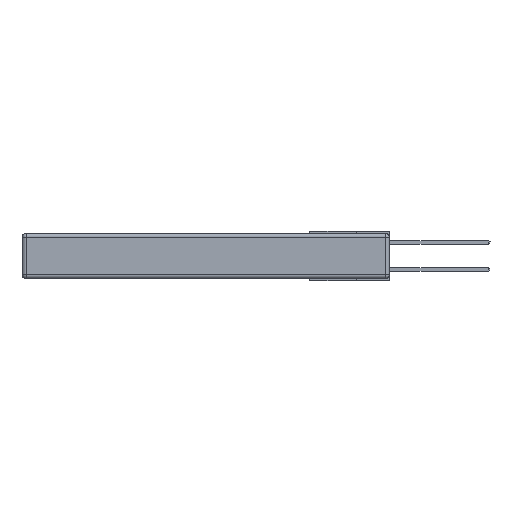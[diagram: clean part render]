
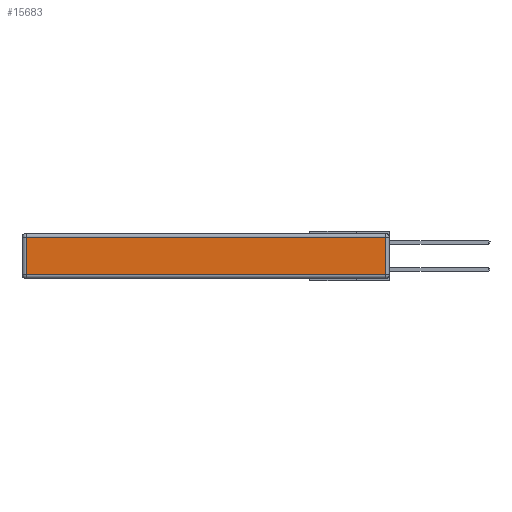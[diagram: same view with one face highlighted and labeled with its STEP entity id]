
A CAD part, left-side view. The second image highlights one B-rep face of the part: STEP entity #15683.
In plain terms, the highlighted planar face has unit normal (-1, 0, 0).
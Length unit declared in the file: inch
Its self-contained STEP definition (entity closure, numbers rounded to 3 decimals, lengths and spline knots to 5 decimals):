
#315 = DIRECTION ( 'NONE',  ( -1., 0., 0. ) ) ;
#1151 = EDGE_CURVE ( 'NONE', #24985, #11487, #11286, .T. ) ;
#1831 = EDGE_LOOP ( 'NONE', ( #15404, #2251, #17438, #33896 ) ) ;
#2251 = ORIENTED_EDGE ( 'NONE', *, *, #24289, .T. ) ;
#4207 = CARTESIAN_POINT ( 'NONE',  ( 0., 0.03, -0.343 ) ) ;
#9116 = VECTOR ( 'NONE', #14674, 39.37008 ) ;
#9779 = CARTESIAN_POINT ( 'NONE',  ( 0., 0.03, -0.313 ) ) ;
#10924 = CARTESIAN_POINT ( 'NONE',  ( 0., 2.72, -0.313 ) ) ;
#11286 = LINE ( 'NONE', #31019, #25665 ) ;
#11487 = VERTEX_POINT ( 'NONE', #10924 ) ;
#13388 = PLANE ( 'NONE',  #25601 ) ;
#13466 = VECTOR ( 'NONE', #32977, 39.37008 ) ;
#13574 = LINE ( 'NONE', #4207, #9116 ) ;
#14564 = CARTESIAN_POINT ( 'NONE',  ( 0., 2.75, -0.03 ) ) ;
#14674 = DIRECTION ( 'NONE',  ( 0., 0., 1. ) ) ;
#14820 = EDGE_CURVE ( 'NONE', #11487, #16382, #22556, .T. ) ;
#15404 = ORIENTED_EDGE ( 'NONE', *, *, #14820, .T. ) ;
#15683 = ADVANCED_FACE ( 'NONE', ( #31113 ), #13388, .T. ) ;
#16382 = VERTEX_POINT ( 'NONE', #9779 ) ;
#17438 = ORIENTED_EDGE ( 'NONE', *, *, #24334, .T. ) ;
#18681 = DIRECTION ( 'NONE',  ( 0., 0., 1. ) ) ;
#22461 = CARTESIAN_POINT ( 'NONE',  ( 0., 0., -0.313 ) ) ;
#22556 = LINE ( 'NONE', #22461, #13466 ) ;
#23064 = VERTEX_POINT ( 'NONE', #25966 ) ;
#23180 = DIRECTION ( 'NONE',  ( 0., 0., -1. ) ) ;
#24289 = EDGE_CURVE ( 'NONE', #16382, #23064, #13574, .T. ) ;
#24332 = LINE ( 'NONE', #14564, #26812 ) ;
#24334 = EDGE_CURVE ( 'NONE', #23064, #24985, #24332, .T. ) ;
#24985 = VERTEX_POINT ( 'NONE', #26198 ) ;
#25601 = AXIS2_PLACEMENT_3D ( 'NONE', #31855, #315, #18681 ) ;
#25665 = VECTOR ( 'NONE', #23180, 39.37008 ) ;
#25966 = CARTESIAN_POINT ( 'NONE',  ( 0., 0.03, -0.03 ) ) ;
#26198 = CARTESIAN_POINT ( 'NONE',  ( 0., 2.72, -0.03 ) ) ;
#26812 = VECTOR ( 'NONE', #28067, 39.37008 ) ;
#28067 = DIRECTION ( 'NONE',  ( 0., 1., 0. ) ) ;
#31019 = CARTESIAN_POINT ( 'NONE',  ( 0., 2.72, -0.343 ) ) ;
#31113 = FACE_OUTER_BOUND ( 'NONE', #1831, .T. ) ;
#31855 = CARTESIAN_POINT ( 'NONE',  ( 0., 0., -0.343 ) ) ;
#32977 = DIRECTION ( 'NONE',  ( 0., -1., 0. ) ) ;
#33896 = ORIENTED_EDGE ( 'NONE', *, *, #1151, .T. ) ;
